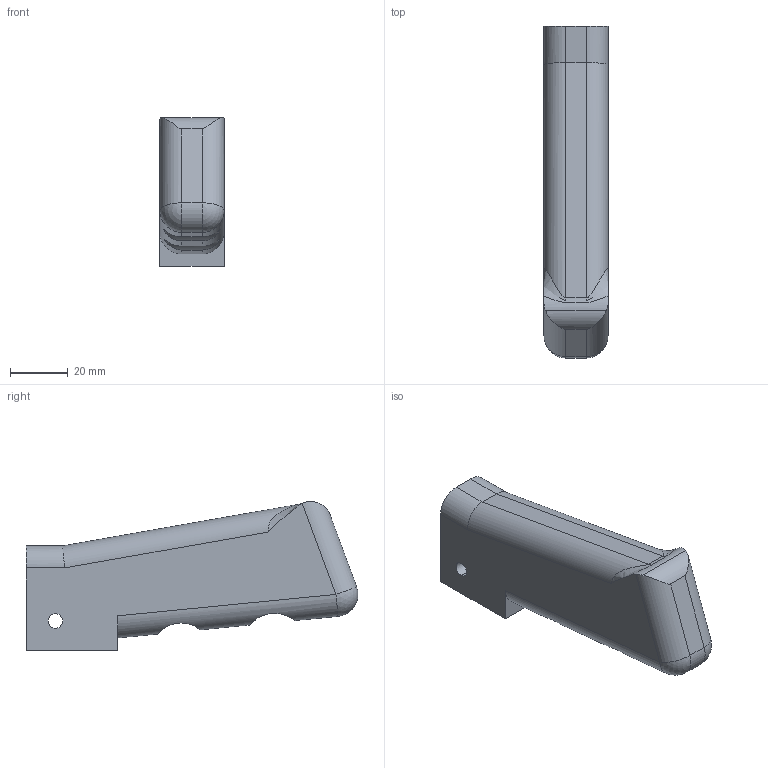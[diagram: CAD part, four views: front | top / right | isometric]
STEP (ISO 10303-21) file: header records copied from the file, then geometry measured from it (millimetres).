
FILE_DESCRIPTION (( 'STEP AP214' ), '1' );
FILE_NAME ('410grip.STEP', '2013-07-25T16:58:30', ( '' ), ( '' ), 'SwSTEP 2.0', 'SolidWorks 2013', '' );
FILE_SCHEMA (( 'AUTOMOTIVE_DESIGN' ));
Length unit declared in the file: inch
Products named in the file (1): 410grip
Bounding box: 22.23 x 114.94 x 51.56 mm (x, y, z)
Volume: 80733.2 mm3; surface area: 14692.4 mm2
Topology: 1 solids, 1 shells, 40 faces, 108 edges, 68 vertices
Faces by surface type: cylinder 20, plane 16, bspline 2, sphere 2
Entity records: 1779 total; most frequent: CARTESIAN_POINT 790, ORIENTED_EDGE 208, DIRECTION 180, EDGE_CURVE 104, VERTEX_POINT 66, LINE 62, VECTOR 62, AXIS2_PLACEMENT_3D 59
